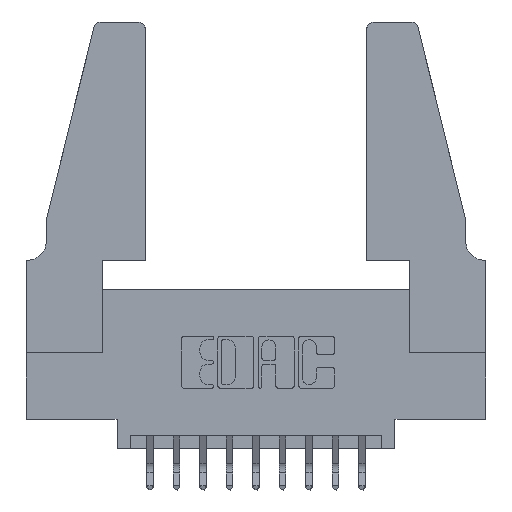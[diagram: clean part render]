
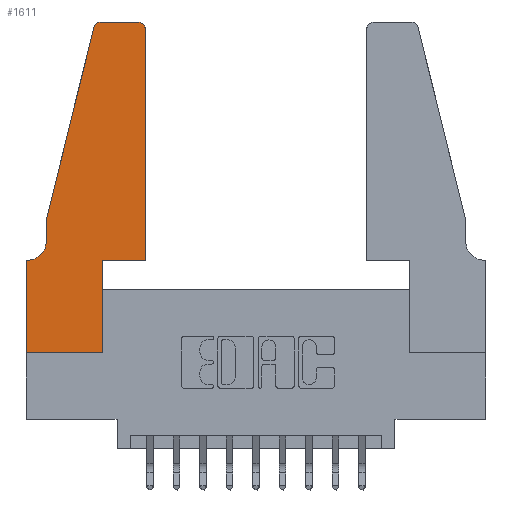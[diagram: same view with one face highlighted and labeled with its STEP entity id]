
A CAD part, top view. The second image highlights one B-rep face of the part: STEP entity #1611.
In plain terms, the highlighted planar face has unit normal (0, 0, 1).
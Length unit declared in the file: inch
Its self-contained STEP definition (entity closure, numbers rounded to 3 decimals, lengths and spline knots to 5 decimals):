
#198 = CARTESIAN_POINT ( 'NONE',  ( 0.284, 1.25, 0.37 ) ) ;
#204 = VERTEX_POINT ( 'NONE', #11472 ) ;
#244 = VERTEX_POINT ( 'NONE', #12501 ) ;
#274 = VERTEX_POINT ( 'NONE', #5331 ) ;
#293 = DIRECTION ( 'NONE',  ( 0., -1., 0. ) ) ;
#582 = DIRECTION ( 'NONE',  ( 0., 1., 0. ) ) ;
#833 = CARTESIAN_POINT ( 'NONE',  ( 0.2865, 0., 0.37 ) ) ;
#856 = DIRECTION ( 'NONE',  ( 0., 0., 1. ) ) ;
#889 = LINE ( 'NONE', #11327, #10199 ) ;
#1068 = CARTESIAN_POINT ( 'NONE',  ( 0., 0., 0.37 ) ) ;
#1391 = EDGE_CURVE ( 'NONE', #9447, #8340, #889, .T. ) ;
#1531 = LINE ( 'NONE', #1991, #10854 ) ;
#1611 = ADVANCED_FACE ( 'NONE', ( #13584 ), #3955, .T. ) ;
#1663 = CIRCLE ( 'NONE', #8191, 0.03 ) ;
#1924 = ORIENTED_EDGE ( 'NONE', *, *, #11647, .T. ) ;
#1991 = CARTESIAN_POINT ( 'NONE',  ( 0.4505, 0.35, 0.37 ) ) ;
#2297 = CARTESIAN_POINT ( 'NONE',  ( 0., 0.35, 0.37 ) ) ;
#2306 = CARTESIAN_POINT ( 'NONE',  ( 0.0755, 0.5, 0.37 ) ) ;
#2310 = DIRECTION ( 'NONE',  ( 0., -1., 0. ) ) ;
#2344 = VERTEX_POINT ( 'NONE', #2297 ) ;
#2518 = VECTOR ( 'NONE', #6505, 39.37008 ) ;
#2697 = ORIENTED_EDGE ( 'NONE', *, *, #5280, .T. ) ;
#2965 = VERTEX_POINT ( 'NONE', #12293 ) ;
#3085 = DIRECTION ( 'NONE',  ( -1., 0., 0. ) ) ;
#3181 = DIRECTION ( 'NONE',  ( 1., 0., 0. ) ) ;
#3361 = CARTESIAN_POINT ( 'NONE',  ( 0.4505, 0.35, 0.37 ) ) ;
#3653 = LINE ( 'NONE', #12780, #6184 ) ;
#3743 = LINE ( 'NONE', #1068, #2518 ) ;
#3856 = ORIENTED_EDGE ( 'NONE', *, *, #6841, .T. ) ;
#3955 = PLANE ( 'NONE',  #11933 ) ;
#4082 = VERTEX_POINT ( 'NONE', #5193 ) ;
#4250 = ORIENTED_EDGE ( 'NONE', *, *, #8269, .T. ) ;
#4597 = CIRCLE ( 'NONE', #12470, 0.07 ) ;
#4663 = AXIS2_PLACEMENT_3D ( 'NONE', #5153, #10442, #7230 ) ;
#4687 = CARTESIAN_POINT ( 'NONE',  ( 0.0755, 0.35, 0.37 ) ) ;
#4751 = DIRECTION ( 'NONE',  ( 0., 0., 1. ) ) ;
#4874 = CARTESIAN_POINT ( 'NONE',  ( 0.2865, 0.35, 0.37 ) ) ;
#5080 = VERTEX_POINT ( 'NONE', #11237 ) ;
#5153 = CARTESIAN_POINT ( 'NONE',  ( 0.4205, 1.22, 0.37 ) ) ;
#5165 = VERTEX_POINT ( 'NONE', #2306 ) ;
#5193 = CARTESIAN_POINT ( 'NONE',  ( 0.4505, 0.35, 0.37 ) ) ;
#5280 = EDGE_CURVE ( 'NONE', #8257, #2965, #1663, .T. ) ;
#5331 = CARTESIAN_POINT ( 'NONE',  ( 0.4505, 1.22, 0.37 ) ) ;
#5935 = ORIENTED_EDGE ( 'NONE', *, *, #7828, .T. ) ;
#5976 = DIRECTION ( 'NONE',  ( 1., 0., 0. ) ) ;
#6184 = VECTOR ( 'NONE', #3085, 39.37008 ) ;
#6244 = CARTESIAN_POINT ( 'NONE',  ( 0.0755, 0.5, 0.37 ) ) ;
#6412 = VECTOR ( 'NONE', #9935, 39.37008 ) ;
#6505 = DIRECTION ( 'NONE',  ( 1., 0., 0. ) ) ;
#6729 = EDGE_CURVE ( 'NONE', #244, #8257, #3653, .T. ) ;
#6841 = EDGE_CURVE ( 'NONE', #204, #2344, #8416, .T. ) ;
#7189 = VECTOR ( 'NONE', #293, 39.37008 ) ;
#7230 = DIRECTION ( 'NONE',  ( 1., 0., 0. ) ) ;
#7824 = CARTESIAN_POINT ( 'NONE',  ( 0.0755, 0.5, 0.37 ) ) ;
#7828 = EDGE_CURVE ( 'NONE', #2344, #5080, #11615, .T. ) ;
#8013 = DIRECTION ( 'NONE',  ( 0., 0., -1. ) ) ;
#8025 = VERTEX_POINT ( 'NONE', #9766 ) ;
#8080 = EDGE_CURVE ( 'NONE', #5165, #8025, #8702, .T. ) ;
#8121 = DIRECTION ( 'NONE',  ( -1., 0., 0. ) ) ;
#8191 = AXIS2_PLACEMENT_3D ( 'NONE', #11350, #4751, #5976 ) ;
#8257 = VERTEX_POINT ( 'NONE', #198 ) ;
#8269 = EDGE_CURVE ( 'NONE', #8025, #204, #4597, .T. ) ;
#8340 = VERTEX_POINT ( 'NONE', #4874 ) ;
#8416 = LINE ( 'NONE', #4687, #9898 ) ;
#8517 = ORIENTED_EDGE ( 'NONE', *, *, #12680, .T. ) ;
#8702 = LINE ( 'NONE', #7824, #8862 ) ;
#8862 = VECTOR ( 'NONE', #2310, 39.37008 ) ;
#9079 = EDGE_CURVE ( 'NONE', #2965, #5165, #9182, .T. ) ;
#9100 = EDGE_CURVE ( 'NONE', #8340, #4082, #1531, .T. ) ;
#9164 = CARTESIAN_POINT ( 'NONE',  ( 0.0055, 0.42, 0.37 ) ) ;
#9182 = LINE ( 'NONE', #6244, #12385 ) ;
#9315 = LINE ( 'NONE', #3361, #6412 ) ;
#9447 = VERTEX_POINT ( 'NONE', #833 ) ;
#9576 = DIRECTION ( 'NONE',  ( -0.239, -0.971, 0. ) ) ;
#9766 = CARTESIAN_POINT ( 'NONE',  ( 0.0755, 0.42, 0.37 ) ) ;
#9898 = VECTOR ( 'NONE', #8121, 39.37008 ) ;
#9935 = DIRECTION ( 'NONE',  ( 0., 1., 0. ) ) ;
#10003 = CARTESIAN_POINT ( 'NONE',  ( 0., 0., 0.37 ) ) ;
#10188 = DIRECTION ( 'NONE',  ( -1., 0., 0. ) ) ;
#10199 = VECTOR ( 'NONE', #582, 39.37008 ) ;
#10442 = DIRECTION ( 'NONE',  ( 0., 0., 1. ) ) ;
#10757 = ORIENTED_EDGE ( 'NONE', *, *, #1391, .T. ) ;
#10798 = ORIENTED_EDGE ( 'NONE', *, *, #6729, .T. ) ;
#10801 = ORIENTED_EDGE ( 'NONE', *, *, #9079, .T. ) ;
#10854 = VECTOR ( 'NONE', #3181, 39.37008 ) ;
#11237 = CARTESIAN_POINT ( 'NONE',  ( 0., 0., 0.37 ) ) ;
#11327 = CARTESIAN_POINT ( 'NONE',  ( 0.2865, 0.35, 0.37 ) ) ;
#11350 = CARTESIAN_POINT ( 'NONE',  ( 0.284, 1.22, 0.37 ) ) ;
#11472 = CARTESIAN_POINT ( 'NONE',  ( 0.0055, 0.35, 0.37 ) ) ;
#11485 = ORIENTED_EDGE ( 'NONE', *, *, #8080, .T. ) ;
#11615 = LINE ( 'NONE', #10003, #7189 ) ;
#11647 = EDGE_CURVE ( 'NONE', #5080, #9447, #3743, .T. ) ;
#11856 = EDGE_LOOP ( 'NONE', ( #10798, #2697, #10801, #11485, #4250, #3856, #5935, #1924, #10757, #13180, #8517, #13614 ) ) ;
#11911 = EDGE_CURVE ( 'NONE', #274, #244, #13051, .T. ) ;
#11933 = AXIS2_PLACEMENT_3D ( 'NONE', #13694, #856, #12745 ) ;
#12293 = CARTESIAN_POINT ( 'NONE',  ( 0.25487, 1.22718, 0.37 ) ) ;
#12385 = VECTOR ( 'NONE', #9576, 39.37008 ) ;
#12470 = AXIS2_PLACEMENT_3D ( 'NONE', #9164, #8013, #10188 ) ;
#12501 = CARTESIAN_POINT ( 'NONE',  ( 0.4205, 1.25, 0.37 ) ) ;
#12680 = EDGE_CURVE ( 'NONE', #4082, #274, #9315, .T. ) ;
#12745 = DIRECTION ( 'NONE',  ( 1., 0., 0. ) ) ;
#12780 = CARTESIAN_POINT ( 'NONE',  ( 0.2605, 1.25, 0.37 ) ) ;
#13051 = CIRCLE ( 'NONE', #4663, 0.03 ) ;
#13180 = ORIENTED_EDGE ( 'NONE', *, *, #9100, .T. ) ;
#13584 = FACE_OUTER_BOUND ( 'NONE', #11856, .T. ) ;
#13614 = ORIENTED_EDGE ( 'NONE', *, *, #11911, .T. ) ;
#13694 = CARTESIAN_POINT ( 'NONE',  ( 0., 0.35, 0.37 ) ) ;
